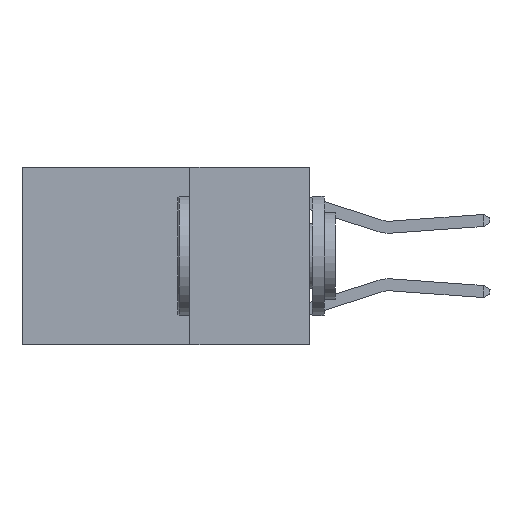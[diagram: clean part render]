
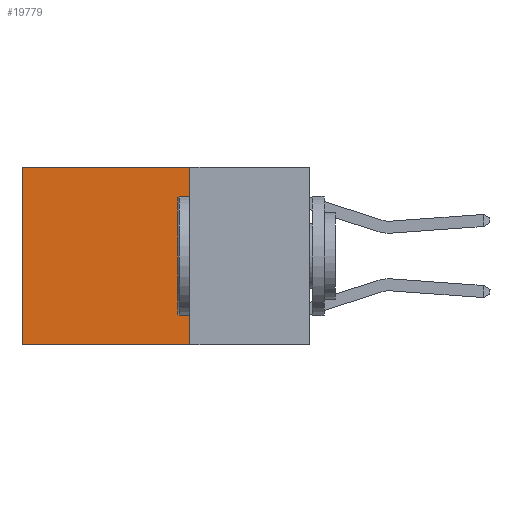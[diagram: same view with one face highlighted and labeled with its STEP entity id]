
A CAD part, left-side view. The second image highlights one B-rep face of the part: STEP entity #19779.
In plain terms, the highlighted planar face has unit normal (-1, 0, 0).
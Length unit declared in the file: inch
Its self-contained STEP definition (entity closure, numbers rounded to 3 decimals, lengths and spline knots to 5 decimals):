
#800 = DIRECTION ( 'NONE',  ( 0., 1., 0. ) ) ;
#1088 = ORIENTED_EDGE ( 'NONE', *, *, #11244, .F. ) ;
#1484 = CARTESIAN_POINT ( 'NONE',  ( 0.2625, 0.25, 0. ) ) ;
#2376 = VERTEX_POINT ( 'NONE', #12591 ) ;
#2751 = DIRECTION ( 'NONE',  ( 0., 0., -1. ) ) ;
#2934 = VERTEX_POINT ( 'NONE', #8215 ) ;
#4591 = DIRECTION ( 'NONE',  ( 1., 0., 0. ) ) ;
#4828 = CARTESIAN_POINT ( 'NONE',  ( 0.2625, 0.25, 0. ) ) ;
#5433 = CARTESIAN_POINT ( 'NONE',  ( 0.2625, 0.25, -0.37 ) ) ;
#7008 = EDGE_CURVE ( 'NONE', #25598, #2376, #8965, .T. ) ;
#7114 = LINE ( 'NONE', #1484, #14177 ) ;
#7677 = ORIENTED_EDGE ( 'NONE', *, *, #31959, .F. ) ;
#8215 = CARTESIAN_POINT ( 'NONE',  ( 0.2625, 0.25, -0.37 ) ) ;
#8965 = LINE ( 'NONE', #14123, #23358 ) ;
#9475 = CARTESIAN_POINT ( 'NONE',  ( 0.2625, 0.25, 0. ) ) ;
#11244 = EDGE_CURVE ( 'NONE', #2934, #2376, #23192, .T. ) ;
#12464 = DIRECTION ( 'NONE',  ( 0., 1., 0. ) ) ;
#12591 = CARTESIAN_POINT ( 'NONE',  ( 0.2625, 0.6, -0.37 ) ) ;
#14123 = CARTESIAN_POINT ( 'NONE',  ( 0.2625, 0.6, 0. ) ) ;
#14177 = VECTOR ( 'NONE', #31848, 39.37008 ) ;
#14283 = DIRECTION ( 'NONE',  ( 0., 0., -1. ) ) ;
#16466 = VECTOR ( 'NONE', #800, 39.37008 ) ;
#16891 = VECTOR ( 'NONE', #12464, 39.37008 ) ;
#17492 = EDGE_CURVE ( 'NONE', #28209, #25598, #17760, .T. ) ;
#17760 = LINE ( 'NONE', #4828, #16891 ) ;
#17852 = CARTESIAN_POINT ( 'NONE',  ( 0.2625, 0.6, 0. ) ) ;
#18276 = ORIENTED_EDGE ( 'NONE', *, *, #17492, .T. ) ;
#19779 = ADVANCED_FACE ( 'NONE', ( #25001 ), #20188, .F. ) ;
#20188 = PLANE ( 'NONE',  #31737 ) ;
#21707 = EDGE_LOOP ( 'NONE', ( #27669, #1088, #7677, #18276 ) ) ;
#23192 = LINE ( 'NONE', #5433, #16466 ) ;
#23358 = VECTOR ( 'NONE', #14283, 39.37008 ) ;
#25001 = FACE_OUTER_BOUND ( 'NONE', #21707, .T. ) ;
#25598 = VERTEX_POINT ( 'NONE', #17852 ) ;
#27669 = ORIENTED_EDGE ( 'NONE', *, *, #7008, .T. ) ;
#28209 = VERTEX_POINT ( 'NONE', #9475 ) ;
#30006 = CARTESIAN_POINT ( 'NONE',  ( 0.2625, 0.25, 0. ) ) ;
#31737 = AXIS2_PLACEMENT_3D ( 'NONE', #30006, #4591, #2751 ) ;
#31848 = DIRECTION ( 'NONE',  ( 0., 0., -1. ) ) ;
#31959 = EDGE_CURVE ( 'NONE', #28209, #2934, #7114, .T. ) ;
